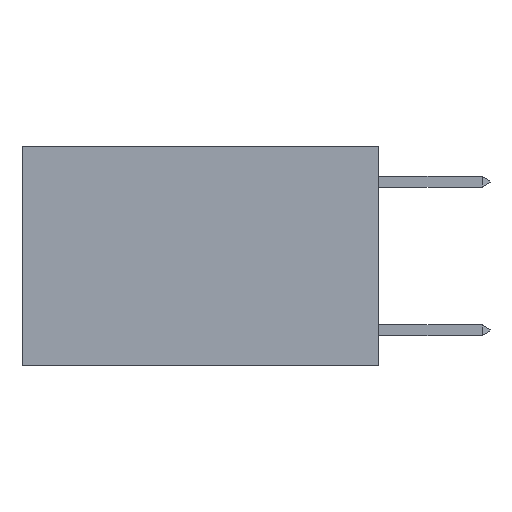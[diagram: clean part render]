
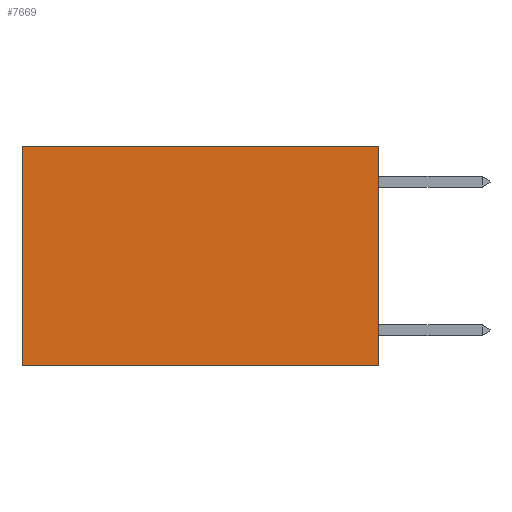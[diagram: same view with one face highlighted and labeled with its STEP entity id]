
A CAD part, left-side view. The second image highlights one B-rep face of the part: STEP entity #7669.
In plain terms, the highlighted planar face has unit normal (-1, 0, 0).
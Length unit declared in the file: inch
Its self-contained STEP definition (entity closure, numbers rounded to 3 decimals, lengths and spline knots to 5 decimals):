
#98 = CARTESIAN_POINT ( 'NONE',  ( 0.2625, 0., 0. ) ) ;
#908 = CARTESIAN_POINT ( 'NONE',  ( 0.2625, 0.6, 0. ) ) ;
#1325 = EDGE_LOOP ( 'NONE', ( #9791, #9948, #2998, #6021 ) ) ;
#1677 = CARTESIAN_POINT ( 'NONE',  ( 0.2625, 0., -0.37 ) ) ;
#1730 = PLANE ( 'NONE',  #9822 ) ;
#1950 = VERTEX_POINT ( 'NONE', #6272 ) ;
#1951 = LINE ( 'NONE', #7120, #2755 ) ;
#2685 = DIRECTION ( 'NONE',  ( 0., 1., 0. ) ) ;
#2755 = VECTOR ( 'NONE', #2685, 39.37008 ) ;
#2998 = ORIENTED_EDGE ( 'NONE', *, *, #5421, .F. ) ;
#3078 = VERTEX_POINT ( 'NONE', #5244 ) ;
#3282 = CARTESIAN_POINT ( 'NONE',  ( 0.2625, 0., 0. ) ) ;
#3451 = DIRECTION ( 'NONE',  ( 1., 0., 0. ) ) ;
#3603 = DIRECTION ( 'NONE',  ( 0., 0., -1. ) ) ;
#4090 = VECTOR ( 'NONE', #9363, 39.37008 ) ;
#4216 = LINE ( 'NONE', #3282, #4090 ) ;
#4320 = DIRECTION ( 'NONE',  ( 0., 0., -1. ) ) ;
#4597 = VECTOR ( 'NONE', #3603, 39.37008 ) ;
#4712 = EDGE_CURVE ( 'NONE', #3078, #5599, #8279, .T. ) ;
#5244 = CARTESIAN_POINT ( 'NONE',  ( 0.2625, 0., 0. ) ) ;
#5421 = EDGE_CURVE ( 'NONE', #3078, #9143, #4216, .T. ) ;
#5599 = VERTEX_POINT ( 'NONE', #9892 ) ;
#6021 = ORIENTED_EDGE ( 'NONE', *, *, #4712, .T. ) ;
#6272 = CARTESIAN_POINT ( 'NONE',  ( 0.2625, 0.6, -0.37 ) ) ;
#6432 = EDGE_CURVE ( 'NONE', #9143, #1950, #1951, .T. ) ;
#6478 = EDGE_CURVE ( 'NONE', #5599, #1950, #7061, .T. ) ;
#7061 = LINE ( 'NONE', #908, #4597 ) ;
#7120 = CARTESIAN_POINT ( 'NONE',  ( 0.2625, 0., -0.37 ) ) ;
#7669 = ADVANCED_FACE ( 'NONE', ( #8622 ), #1730, .F. ) ;
#8279 = LINE ( 'NONE', #10725, #10014 ) ;
#8622 = FACE_OUTER_BOUND ( 'NONE', #1325, .T. ) ;
#9143 = VERTEX_POINT ( 'NONE', #1677 ) ;
#9363 = DIRECTION ( 'NONE',  ( 0., 0., -1. ) ) ;
#9791 = ORIENTED_EDGE ( 'NONE', *, *, #6478, .T. ) ;
#9822 = AXIS2_PLACEMENT_3D ( 'NONE', #98, #3451, #4320 ) ;
#9892 = CARTESIAN_POINT ( 'NONE',  ( 0.2625, 0.6, 0. ) ) ;
#9948 = ORIENTED_EDGE ( 'NONE', *, *, #6432, .F. ) ;
#10014 = VECTOR ( 'NONE', #10043, 39.37008 ) ;
#10043 = DIRECTION ( 'NONE',  ( 0., 1., 0. ) ) ;
#10725 = CARTESIAN_POINT ( 'NONE',  ( 0.2625, 0., 0. ) ) ;
